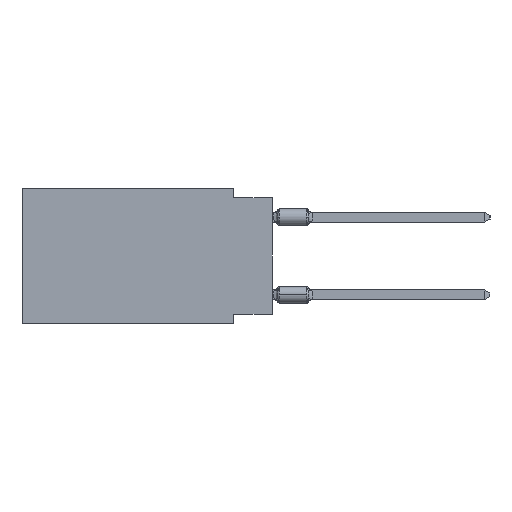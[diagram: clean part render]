
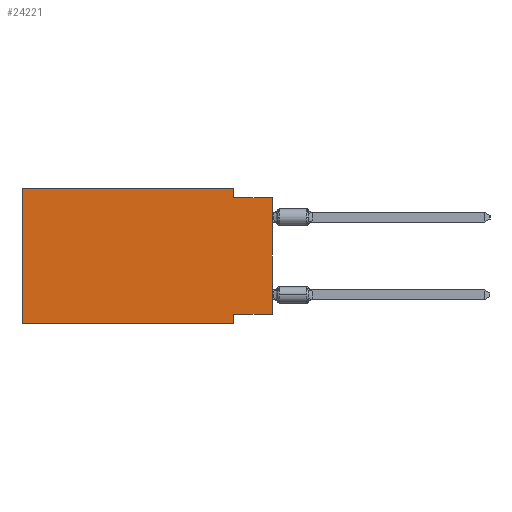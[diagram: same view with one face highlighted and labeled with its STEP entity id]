
A CAD part, left-side view. The second image highlights one B-rep face of the part: STEP entity #24221.
In plain terms, the highlighted planar face has unit normal (-1, 0, 0).
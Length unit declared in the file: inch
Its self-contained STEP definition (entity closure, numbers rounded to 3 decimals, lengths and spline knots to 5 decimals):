
#438 = ORIENTED_EDGE ( 'NONE', *, *, #15592, .F. ) ;
#477 = ORIENTED_EDGE ( 'NONE', *, *, #27659, .F. ) ;
#1414 = FACE_OUTER_BOUND ( 'NONE', #12640, .T. ) ;
#1893 = VERTEX_POINT ( 'NONE', #10344 ) ;
#2086 = CARTESIAN_POINT ( 'NONE',  ( 0., 0.1, -0.35 ) ) ;
#3391 = VERTEX_POINT ( 'NONE', #2086 ) ;
#4121 = VECTOR ( 'NONE', #8809, 39.37008 ) ;
#4645 = CARTESIAN_POINT ( 'NONE',  ( 0., 0.645, -0.35 ) ) ;
#4910 = CARTESIAN_POINT ( 'NONE',  ( 0., 0.1, -0.35 ) ) ;
#4953 = LINE ( 'NONE', #13672, #19409 ) ;
#5123 = EDGE_CURVE ( 'NONE', #7696, #19576, #24907, .T. ) ;
#5193 = DIRECTION ( 'NONE',  ( 0., -1., 0. ) ) ;
#5646 = DIRECTION ( 'NONE',  ( 0., 0., 1. ) ) ;
#6135 = ORIENTED_EDGE ( 'NONE', *, *, #5123, .T. ) ;
#6177 = LINE ( 'NONE', #6453, #16698 ) ;
#6274 = EDGE_CURVE ( 'NONE', #17263, #3391, #24167, .T. ) ;
#6453 = CARTESIAN_POINT ( 'NONE',  ( 0., 0.645, 0. ) ) ;
#6508 = AXIS2_PLACEMENT_3D ( 'NONE', #23079, #14233, #26895 ) ;
#6849 = VECTOR ( 'NONE', #5193, 39.37008 ) ;
#6895 = LINE ( 'NONE', #4645, #6849 ) ;
#7074 = DIRECTION ( 'NONE',  ( 0., 0., -1. ) ) ;
#7696 = VERTEX_POINT ( 'NONE', #24549 ) ;
#7872 = ORIENTED_EDGE ( 'NONE', *, *, #19374, .F. ) ;
#7992 = ORIENTED_EDGE ( 'NONE', *, *, #16746, .F. ) ;
#8150 = VECTOR ( 'NONE', #18333, 39.37008 ) ;
#8703 = DIRECTION ( 'NONE',  ( 0., 0., 1. ) ) ;
#8809 = DIRECTION ( 'NONE',  ( 0., -1., 0. ) ) ;
#9676 = ORIENTED_EDGE ( 'NONE', *, *, #17243, .T. ) ;
#10002 = VERTEX_POINT ( 'NONE', #19672 ) ;
#10071 = LINE ( 'NONE', #14144, #14404 ) ;
#10344 = CARTESIAN_POINT ( 'NONE',  ( 0., 0.645, 0. ) ) ;
#10871 = CARTESIAN_POINT ( 'NONE',  ( 0., 0.1, 0. ) ) ;
#11070 = ORIENTED_EDGE ( 'NONE', *, *, #6274, .F. ) ;
#12640 = EDGE_LOOP ( 'NONE', ( #6135, #7872, #477, #438, #7992, #9676, #11070, #15424 ) ) ;
#13340 = EDGE_CURVE ( 'NONE', #7696, #17263, #10071, .T. ) ;
#13398 = VECTOR ( 'NONE', #21769, 39.37008 ) ;
#13672 = CARTESIAN_POINT ( 'NONE',  ( 0., 0.1, 0. ) ) ;
#14144 = CARTESIAN_POINT ( 'NONE',  ( 0., 0., -0.325 ) ) ;
#14233 = DIRECTION ( 'NONE',  ( 1., 0., 0. ) ) ;
#14404 = VECTOR ( 'NONE', #27107, 39.37008 ) ;
#15408 = CARTESIAN_POINT ( 'NONE',  ( 0., 0., -0.025 ) ) ;
#15424 = ORIENTED_EDGE ( 'NONE', *, *, #13340, .F. ) ;
#15592 = EDGE_CURVE ( 'NONE', #1893, #15826, #22392, .T. ) ;
#15826 = VERTEX_POINT ( 'NONE', #10871 ) ;
#16698 = VECTOR ( 'NONE', #8703, 39.37008 ) ;
#16746 = EDGE_CURVE ( 'NONE', #19458, #1893, #6177, .T. ) ;
#17243 = EDGE_CURVE ( 'NONE', #19458, #3391, #6895, .T. ) ;
#17263 = VERTEX_POINT ( 'NONE', #24028 ) ;
#17351 = LINE ( 'NONE', #15408, #4121 ) ;
#17904 = CARTESIAN_POINT ( 'NONE',  ( 0., 0.645, -0.35 ) ) ;
#18333 = DIRECTION ( 'NONE',  ( 0., -1., 0. ) ) ;
#18769 = CARTESIAN_POINT ( 'NONE',  ( 0., 0., -0.025 ) ) ;
#19374 = EDGE_CURVE ( 'NONE', #10002, #19576, #17351, .T. ) ;
#19409 = VECTOR ( 'NONE', #7074, 39.37008 ) ;
#19458 = VERTEX_POINT ( 'NONE', #17904 ) ;
#19576 = VERTEX_POINT ( 'NONE', #18769 ) ;
#19672 = CARTESIAN_POINT ( 'NONE',  ( 0., 0.1, -0.025 ) ) ;
#20454 = CARTESIAN_POINT ( 'NONE',  ( 0., 0.645, 0. ) ) ;
#21769 = DIRECTION ( 'NONE',  ( 0., 0., -1. ) ) ;
#22392 = LINE ( 'NONE', #20454, #8150 ) ;
#22916 = CARTESIAN_POINT ( 'NONE',  ( 0., 0., 0. ) ) ;
#23079 = CARTESIAN_POINT ( 'NONE',  ( 0., 0.645, 0. ) ) ;
#24028 = CARTESIAN_POINT ( 'NONE',  ( 0., 0.1, -0.325 ) ) ;
#24167 = LINE ( 'NONE', #4910, #13398 ) ;
#24221 = ADVANCED_FACE ( 'NONE', ( #1414 ), #24621, .F. ) ;
#24549 = CARTESIAN_POINT ( 'NONE',  ( 0., 0., -0.325 ) ) ;
#24621 = PLANE ( 'NONE',  #6508 ) ;
#24907 = LINE ( 'NONE', #22916, #27764 ) ;
#26895 = DIRECTION ( 'NONE',  ( 0., 0., -1. ) ) ;
#27107 = DIRECTION ( 'NONE',  ( 0., 1., 0. ) ) ;
#27659 = EDGE_CURVE ( 'NONE', #15826, #10002, #4953, .T. ) ;
#27764 = VECTOR ( 'NONE', #5646, 39.37008 ) ;
